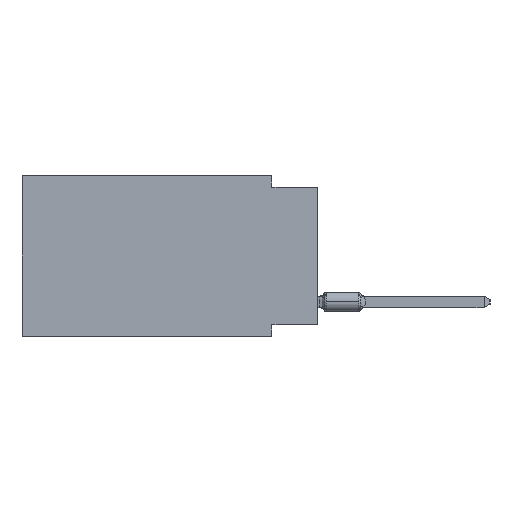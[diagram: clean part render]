
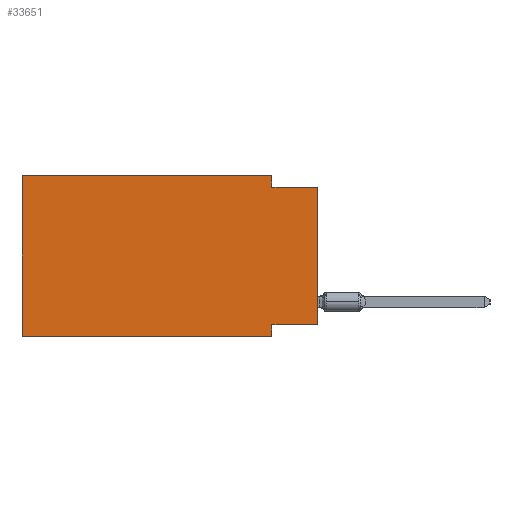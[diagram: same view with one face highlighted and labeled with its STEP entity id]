
A CAD part, left-side view. The second image highlights one B-rep face of the part: STEP entity #33651.
In plain terms, the highlighted planar face has unit normal (-1, 0, 0).
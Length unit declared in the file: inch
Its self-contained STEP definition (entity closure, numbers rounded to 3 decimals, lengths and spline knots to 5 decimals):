
#646 = FACE_OUTER_BOUND ( 'NONE', #20126, .T. ) ;
#829 = ORIENTED_EDGE ( 'NONE', *, *, #31074, .T. ) ;
#1307 = DIRECTION ( 'NONE',  ( 0., 0., -1. ) ) ;
#1581 = ORIENTED_EDGE ( 'NONE', *, *, #8915, .F. ) ;
#1630 = VECTOR ( 'NONE', #1307, 39.37008 ) ;
#1970 = LINE ( 'NONE', #11261, #20703 ) ;
#2505 = VERTEX_POINT ( 'NONE', #22909 ) ;
#2860 = CARTESIAN_POINT ( 'NONE',  ( 0., 0., -0.325 ) ) ;
#2959 = CARTESIAN_POINT ( 'NONE',  ( 0., 0.645, -0.35 ) ) ;
#3778 = CARTESIAN_POINT ( 'NONE',  ( 0., 0.1, -0.325 ) ) ;
#4740 = VERTEX_POINT ( 'NONE', #20698 ) ;
#4845 = EDGE_CURVE ( 'NONE', #31917, #26991, #12567, .T. ) ;
#5353 = VECTOR ( 'NONE', #17898, 39.37008 ) ;
#6388 = EDGE_CURVE ( 'NONE', #30339, #2505, #15114, .T. ) ;
#7590 = LINE ( 'NONE', #36333, #16255 ) ;
#8765 = AXIS2_PLACEMENT_3D ( 'NONE', #23098, #34400, #20310 ) ;
#8915 = EDGE_CURVE ( 'NONE', #31917, #17865, #14311, .T. ) ;
#9040 = LINE ( 'NONE', #2959, #27605 ) ;
#11261 = CARTESIAN_POINT ( 'NONE',  ( 0., 0.1, -0.35 ) ) ;
#11801 = PLANE ( 'NONE',  #8765 ) ;
#12567 = LINE ( 'NONE', #15708, #33188 ) ;
#12575 = CARTESIAN_POINT ( 'NONE',  ( 0., 0.1, -0.025 ) ) ;
#13239 = ORIENTED_EDGE ( 'NONE', *, *, #29051, .F. ) ;
#14277 = DIRECTION ( 'NONE',  ( 0., -1., 0. ) ) ;
#14311 = LINE ( 'NONE', #14846, #26459 ) ;
#14846 = CARTESIAN_POINT ( 'NONE',  ( 0., 0., -0.325 ) ) ;
#15114 = LINE ( 'NONE', #24014, #5353 ) ;
#15708 = CARTESIAN_POINT ( 'NONE',  ( 0., 0., 0. ) ) ;
#16255 = VECTOR ( 'NONE', #30954, 39.37008 ) ;
#17105 = EDGE_CURVE ( 'NONE', #31204, #26991, #7590, .T. ) ;
#17865 = VERTEX_POINT ( 'NONE', #3778 ) ;
#17898 = DIRECTION ( 'NONE',  ( 0., 0., 1. ) ) ;
#18181 = ORIENTED_EDGE ( 'NONE', *, *, #4845, .T. ) ;
#18792 = CARTESIAN_POINT ( 'NONE',  ( 0., 0.645, -0.35 ) ) ;
#19081 = CARTESIAN_POINT ( 'NONE',  ( 0., 0.645, 0. ) ) ;
#20126 = EDGE_LOOP ( 'NONE', ( #18181, #24932, #35525, #13239, #28558, #829, #25389, #1581 ) ) ;
#20310 = DIRECTION ( 'NONE',  ( 0., 0., -1. ) ) ;
#20698 = CARTESIAN_POINT ( 'NONE',  ( 0., 0.1, -0.35 ) ) ;
#20703 = VECTOR ( 'NONE', #27940, 39.37008 ) ;
#20892 = DIRECTION ( 'NONE',  ( 0., 0., 1. ) ) ;
#22909 = CARTESIAN_POINT ( 'NONE',  ( 0., 0.645, 0. ) ) ;
#23098 = CARTESIAN_POINT ( 'NONE',  ( 0., 0.645, 0. ) ) ;
#24014 = CARTESIAN_POINT ( 'NONE',  ( 0., 0.645, 0. ) ) ;
#24130 = CARTESIAN_POINT ( 'NONE',  ( 0., 0.1, 0. ) ) ;
#24932 = ORIENTED_EDGE ( 'NONE', *, *, #17105, .F. ) ;
#25389 = ORIENTED_EDGE ( 'NONE', *, *, #35639, .F. ) ;
#25401 = EDGE_CURVE ( 'NONE', #26487, #31204, #32268, .T. ) ;
#26165 = CARTESIAN_POINT ( 'NONE',  ( 0., 0., -0.025 ) ) ;
#26459 = VECTOR ( 'NONE', #34480, 39.37008 ) ;
#26487 = VERTEX_POINT ( 'NONE', #27962 ) ;
#26702 = VECTOR ( 'NONE', #30369, 39.37008 ) ;
#26991 = VERTEX_POINT ( 'NONE', #26165 ) ;
#27605 = VECTOR ( 'NONE', #14277, 39.37008 ) ;
#27940 = DIRECTION ( 'NONE',  ( 0., 0., -1. ) ) ;
#27962 = CARTESIAN_POINT ( 'NONE',  ( 0., 0.1, 0. ) ) ;
#28558 = ORIENTED_EDGE ( 'NONE', *, *, #6388, .F. ) ;
#29051 = EDGE_CURVE ( 'NONE', #2505, #26487, #34054, .T. ) ;
#30339 = VERTEX_POINT ( 'NONE', #18792 ) ;
#30369 = DIRECTION ( 'NONE',  ( 0., -1., 0. ) ) ;
#30954 = DIRECTION ( 'NONE',  ( 0., -1., 0. ) ) ;
#31074 = EDGE_CURVE ( 'NONE', #30339, #4740, #9040, .T. ) ;
#31204 = VERTEX_POINT ( 'NONE', #12575 ) ;
#31917 = VERTEX_POINT ( 'NONE', #2860 ) ;
#32268 = LINE ( 'NONE', #24130, #1630 ) ;
#33188 = VECTOR ( 'NONE', #20892, 39.37008 ) ;
#33651 = ADVANCED_FACE ( 'NONE', ( #646 ), #11801, .F. ) ;
#34054 = LINE ( 'NONE', #19081, #26702 ) ;
#34400 = DIRECTION ( 'NONE',  ( 1., 0., 0. ) ) ;
#34480 = DIRECTION ( 'NONE',  ( 0., 1., 0. ) ) ;
#35525 = ORIENTED_EDGE ( 'NONE', *, *, #25401, .F. ) ;
#35639 = EDGE_CURVE ( 'NONE', #17865, #4740, #1970, .T. ) ;
#36333 = CARTESIAN_POINT ( 'NONE',  ( 0., 0., -0.025 ) ) ;
